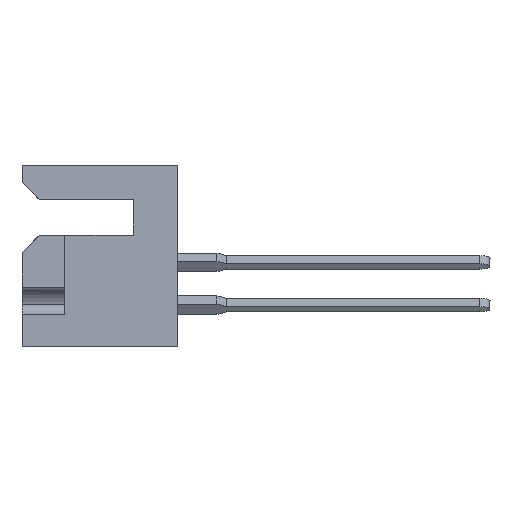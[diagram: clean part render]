
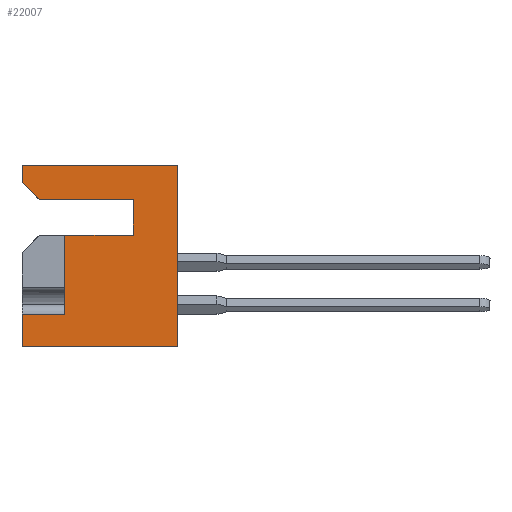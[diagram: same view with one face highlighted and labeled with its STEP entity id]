
A CAD part, left-side view. The second image highlights one B-rep face of the part: STEP entity #22007.
In plain terms, the highlighted planar face has unit normal (-1, 0, 0).
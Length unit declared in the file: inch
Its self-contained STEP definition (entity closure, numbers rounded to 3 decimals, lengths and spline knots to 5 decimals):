
#468 = CARTESIAN_POINT ( 'NONE',  ( 0., 0., 0. ) ) ;
#1963 = DIRECTION ( 'NONE',  ( 1., 0., 0. ) ) ;
#2371 = ORIENTED_EDGE ( 'NONE', *, *, #3402, .F. ) ;
#2409 = EDGE_CURVE ( 'NONE', #8371, #29093, #28460, .T. ) ;
#2677 = VERTEX_POINT ( 'NONE', #26982 ) ;
#2738 = EDGE_CURVE ( 'NONE', #8371, #26145, #17986, .T. ) ;
#2812 = EDGE_LOOP ( 'NONE', ( #17189, #23229, #3385, #25568, #29890, #2371, #29833, #7258, #30213, #27747, #19642 ) ) ;
#3385 = ORIENTED_EDGE ( 'NONE', *, *, #2738, .T. ) ;
#3402 = EDGE_CURVE ( 'NONE', #15600, #28365, #27594, .T. ) ;
#3413 = EDGE_CURVE ( 'NONE', #2677, #30651, #18715, .T. ) ;
#3621 = CARTESIAN_POINT ( 'NONE',  ( 0., 0.128, -0.1 ) ) ;
#4581 = VERTEX_POINT ( 'NONE', #24032 ) ;
#4909 = VERTEX_POINT ( 'NONE', #3621 ) ;
#5320 = EDGE_CURVE ( 'NONE', #4581, #29093, #17494, .T. ) ;
#6179 = CARTESIAN_POINT ( 'NONE',  ( 0., 0.453, -0.531 ) ) ;
#6314 = VECTOR ( 'NONE', #20299, 39.37008 ) ;
#6404 = DIRECTION ( 'NONE',  ( 0., -1., 0. ) ) ;
#7017 = VECTOR ( 'NONE', #13381, 39.37008 ) ;
#7193 = VECTOR ( 'NONE', #12864, 39.37008 ) ;
#7258 = ORIENTED_EDGE ( 'NONE', *, *, #19005, .F. ) ;
#7639 = VECTOR ( 'NONE', #19613, 39.37008 ) ;
#8371 = VERTEX_POINT ( 'NONE', #6179 ) ;
#8603 = VECTOR ( 'NONE', #19887, 39.37008 ) ;
#8619 = CARTESIAN_POINT ( 'NONE',  ( 0., 0.403, -0.1 ) ) ;
#8927 = VECTOR ( 'NONE', #12023, 39.37008 ) ;
#11055 = EDGE_CURVE ( 'NONE', #4581, #30651, #15862, .T. ) ;
#11186 = CARTESIAN_POINT ( 'NONE',  ( 0., 0.453, 0. ) ) ;
#11294 = CARTESIAN_POINT ( 'NONE',  ( 0., 0.128, -0.1 ) ) ;
#12023 = DIRECTION ( 'NONE',  ( 0., -0.707, -0.707 ) ) ;
#12620 = CARTESIAN_POINT ( 'NONE',  ( 0., 0.128, -0.205 ) ) ;
#12864 = DIRECTION ( 'NONE',  ( 0., -1., 0. ) ) ;
#13033 = CARTESIAN_POINT ( 'NONE',  ( 0., 0.328, -0.437 ) ) ;
#13381 = DIRECTION ( 'NONE',  ( 0., 0., 1. ) ) ;
#13592 = DIRECTION ( 'NONE',  ( 0., 0., -1. ) ) ;
#13740 = LINE ( 'NONE', #23441, #28992 ) ;
#14109 = CARTESIAN_POINT ( 'NONE',  ( 0., 0.328, -0.205 ) ) ;
#14533 = CARTESIAN_POINT ( 'NONE',  ( 0., 0.453, 0. ) ) ;
#14661 = EDGE_CURVE ( 'NONE', #26145, #17997, #13740, .T. ) ;
#15600 = VERTEX_POINT ( 'NONE', #20432 ) ;
#15733 = VECTOR ( 'NONE', #22074, 39.37008 ) ;
#15816 = PLANE ( 'NONE',  #28926 ) ;
#15862 = LINE ( 'NONE', #17140, #7639 ) ;
#17140 = CARTESIAN_POINT ( 'NONE',  ( 0., 0.328, -0.205 ) ) ;
#17189 = ORIENTED_EDGE ( 'NONE', *, *, #5320, .T. ) ;
#17494 = LINE ( 'NONE', #13033, #6314 ) ;
#17986 = LINE ( 'NONE', #22320, #7193 ) ;
#17997 = VERTEX_POINT ( 'NONE', #468 ) ;
#18084 = LINE ( 'NONE', #11186, #23650 ) ;
#18715 = LINE ( 'NONE', #12620, #8603 ) ;
#19005 = EDGE_CURVE ( 'NONE', #4909, #26060, #24160, .T. ) ;
#19291 = EDGE_CURVE ( 'NONE', #2677, #4909, #21921, .T. ) ;
#19613 = DIRECTION ( 'NONE',  ( 0., 0., 1. ) ) ;
#19642 = ORIENTED_EDGE ( 'NONE', *, *, #11055, .F. ) ;
#19675 = CARTESIAN_POINT ( 'NONE',  ( 0., 0.453, 0. ) ) ;
#19887 = DIRECTION ( 'NONE',  ( 0., 1., 0. ) ) ;
#20299 = DIRECTION ( 'NONE',  ( 0., 1., 0. ) ) ;
#20432 = CARTESIAN_POINT ( 'NONE',  ( 0., 0.453, -0.05 ) ) ;
#20614 = FACE_OUTER_BOUND ( 'NONE', #2812, .T. ) ;
#21023 = VECTOR ( 'NONE', #25533, 39.37008 ) ;
#21640 = CARTESIAN_POINT ( 'NONE',  ( 0., 0.453, -0.437 ) ) ;
#21921 = LINE ( 'NONE', #11294, #7017 ) ;
#22007 = ADVANCED_FACE ( 'NONE', ( #20614 ), #15816, .F. ) ;
#22074 = DIRECTION ( 'NONE',  ( 0., 0., 1. ) ) ;
#22320 = CARTESIAN_POINT ( 'NONE',  ( 0., 0.453, -0.531 ) ) ;
#23229 = ORIENTED_EDGE ( 'NONE', *, *, #2409, .F. ) ;
#23441 = CARTESIAN_POINT ( 'NONE',  ( 0., 0., 0. ) ) ;
#23476 = LINE ( 'NONE', #26262, #8927 ) ;
#23650 = VECTOR ( 'NONE', #6404, 39.37008 ) ;
#23800 = VECTOR ( 'NONE', #26995, 39.37008 ) ;
#24032 = CARTESIAN_POINT ( 'NONE',  ( 0., 0.328, -0.437 ) ) ;
#24160 = LINE ( 'NONE', #29113, #23800 ) ;
#25533 = DIRECTION ( 'NONE',  ( 0., 0., 1. ) ) ;
#25568 = ORIENTED_EDGE ( 'NONE', *, *, #14661, .T. ) ;
#25795 = CARTESIAN_POINT ( 'NONE',  ( 0., 0., -0.531 ) ) ;
#26060 = VERTEX_POINT ( 'NONE', #8619 ) ;
#26145 = VERTEX_POINT ( 'NONE', #25795 ) ;
#26262 = CARTESIAN_POINT ( 'NONE',  ( 0., 0.403, -0.1 ) ) ;
#26968 = DIRECTION ( 'NONE',  ( 0., 0., 1. ) ) ;
#26982 = CARTESIAN_POINT ( 'NONE',  ( 0., 0.128, -0.205 ) ) ;
#26995 = DIRECTION ( 'NONE',  ( 0., 1., 0. ) ) ;
#27594 = LINE ( 'NONE', #19675, #15733 ) ;
#27747 = ORIENTED_EDGE ( 'NONE', *, *, #3413, .T. ) ;
#27831 = CARTESIAN_POINT ( 'NONE',  ( 0., 0.453, 0. ) ) ;
#28365 = VERTEX_POINT ( 'NONE', #14533 ) ;
#28389 = EDGE_CURVE ( 'NONE', #15600, #26060, #23476, .T. ) ;
#28460 = LINE ( 'NONE', #30231, #21023 ) ;
#28926 = AXIS2_PLACEMENT_3D ( 'NONE', #27831, #1963, #13592 ) ;
#28992 = VECTOR ( 'NONE', #26968, 39.37008 ) ;
#29093 = VERTEX_POINT ( 'NONE', #21640 ) ;
#29113 = CARTESIAN_POINT ( 'NONE',  ( 0., 0.128, -0.1 ) ) ;
#29833 = ORIENTED_EDGE ( 'NONE', *, *, #28389, .T. ) ;
#29890 = ORIENTED_EDGE ( 'NONE', *, *, #29973, .F. ) ;
#29973 = EDGE_CURVE ( 'NONE', #28365, #17997, #18084, .T. ) ;
#30213 = ORIENTED_EDGE ( 'NONE', *, *, #19291, .F. ) ;
#30231 = CARTESIAN_POINT ( 'NONE',  ( 0., 0.453, 0. ) ) ;
#30651 = VERTEX_POINT ( 'NONE', #14109 ) ;
